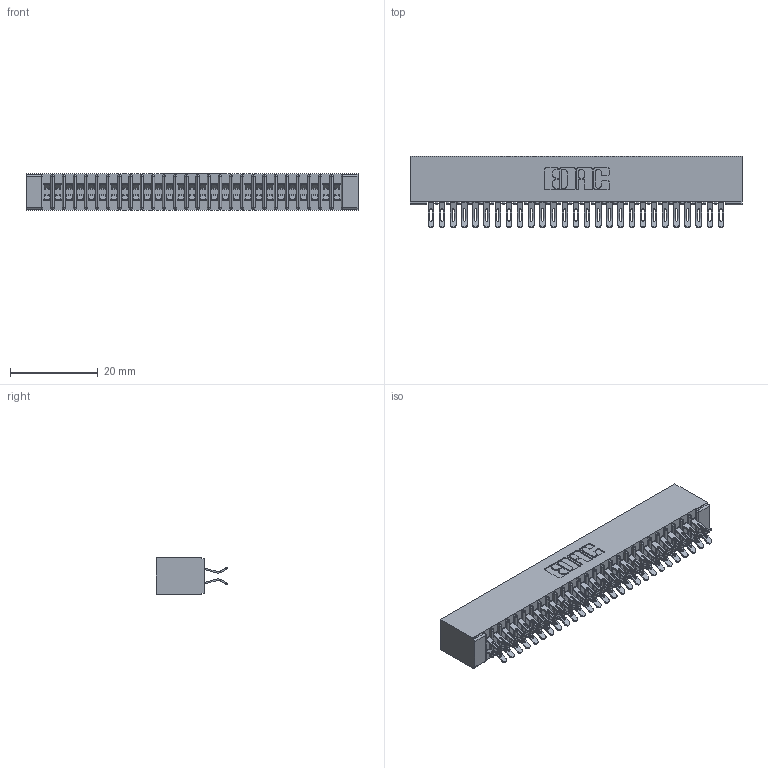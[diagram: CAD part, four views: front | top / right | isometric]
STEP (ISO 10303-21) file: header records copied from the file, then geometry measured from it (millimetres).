
FILE_DESCRIPTION (( 'STEP AP203' ), '1' );
FILE_NAME ('341-054-555-201.STEP', '2018-08-07T14:26:56', ( '' ), ( '' ), 'SwSTEP 2.0', 'SolidWorks 2016', '' );
FILE_SCHEMA (( 'CONFIG_CONTROL_DESIGN' ));
Length unit declared in the file: inch
Products named in the file (3): 341 Part_No Mounting Lugs; 341-292-001_341-292-155; 341-054-555-201
Assembly tree (55 placements, depth 2):
  341-054-555-201
    341 Part_No Mounting Lugs
    341-292-001_341-292-155  x54
Bounding box: 75.56 x 16.31 x 8.38 mm (x, y, z)
Volume: 4485.8 mm3; surface area: 10746.4 mm2
Topology: 55 solids, 55 shells, 4320 faces, 12901 edges, 8398 vertices
Faces by surface type: plane 2332, cylinder 1880, sphere 56, torus 52
Entity records: 34866 total; most frequent: CARTESIAN_POINT 5811, ORIENTED_EDGE 5762, DIRECTION 5639, EDGE_CURVE 2881, VECTOR 2299, LINE 2299, VERTEX_POINT 1826, AXIS2_PLACEMENT_3D 1670
